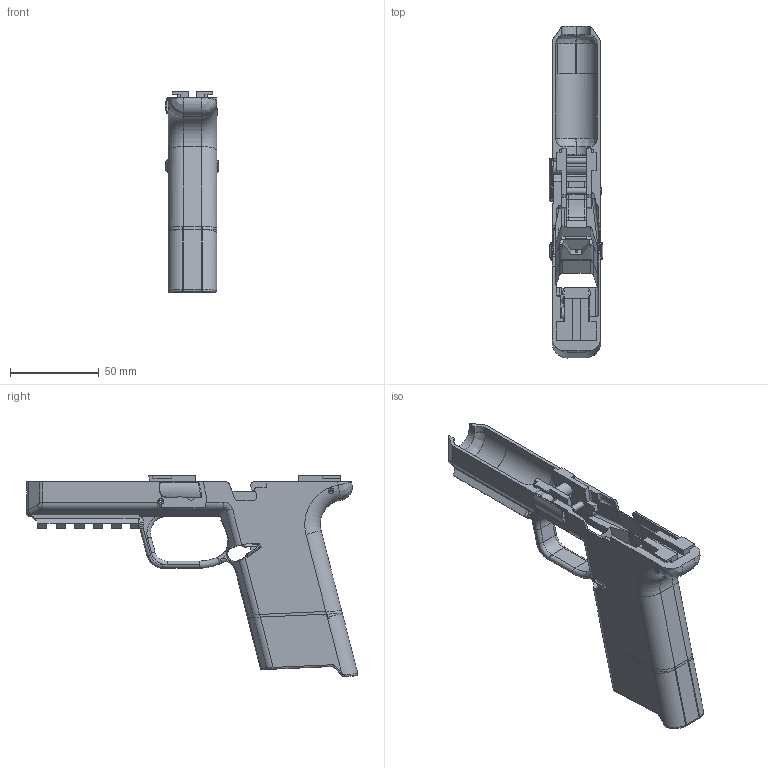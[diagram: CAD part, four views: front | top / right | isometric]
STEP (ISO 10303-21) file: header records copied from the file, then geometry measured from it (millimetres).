
FILE_DESCRIPTION(/* description */ (''),/* implementation_level */ '2;1');
FILE_NAME(/* name */ 'M&P 9 Assembly + Picatinny - Full Size Slide.step',/* time_stamp */ '2021-11-06T19:35:58-04:00',/* author */ (''),/* organization */ (''),/* preprocessor_version */ 'ST-DEVELOPER v18.1',/* originating_system */ 'Autodesk Translation Framework v10.10.0.1391',/* authorisation */ '');
FILE_SCHEMA (('AUTOMOTIVE_DESIGN { 1 0 10303 214 3 1 1 }'));
Length unit declared in the file: millimetre
Products named in the file (13): M&P 9 Standard Length Slide - Picatinny; M&P 9 Reference v102; Rear Fire Control Group Pin; Front Locking Block Group Pin; Trigger Pin; Locking Block; Disassembly Lug; Rear Fire Control Group; Frame; Trigger Guard and Magwell; Fitment Section; Nose; Full-Size Magwell Body
Assembly tree (12 placements, depth 5):
  M&P 9 Standard Length Slide - Picatinny
    M&P 9 Reference v102
      Rear Fire Control Group Pin
      Front Locking Block Group Pin
      Trigger Pin
      Locking Block
      Disassembly Lug
      Rear Fire Control Group
      Frame
        Trigger Guard and Magwell
        Fitment Section
          Nose
        Full-Size Magwell Body
Bounding box: 30.21 x 186.78 x 113.13 mm (x, y, z)
Volume: 106983.2 mm3; surface area: 57862.9 mm2
Topology: 10 solids, 10 shells, 659 faces, 1797 edges, 1144 vertices
Faces by surface type: plane 336, cylinder 197, bspline 100, torus 21, sphere 4, cone 1
Full cylindrical faces by diameter (mm): 1.35 x2, 1.5 x3, 3.15 x2, 3.18 x3, 3.2 x2, 3.361 x2, 3.5 x1, 3.55 x4, 4.7 x2, 6.3 x1, 7.7 x1, 8.8 x1, 9 x2
Entity records: 24224 total; most frequent: CARTESIAN_POINT 7401, ORIENTED_EDGE 3586, DIRECTION 3284, EDGE_CURVE 1793, VERTEX_POINT 1144, AXIS2_PLACEMENT_3D 1098, LINE 1088, VECTOR 1088
